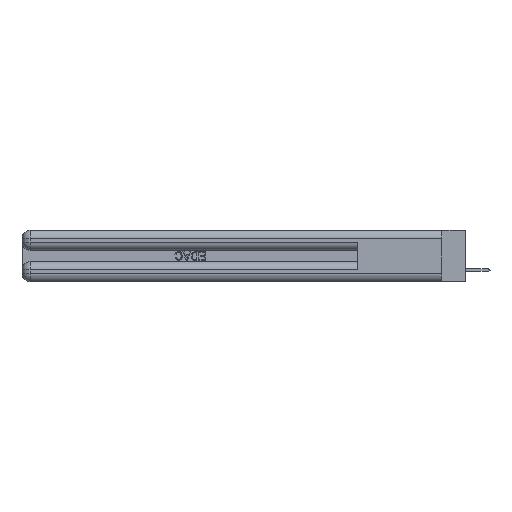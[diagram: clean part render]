
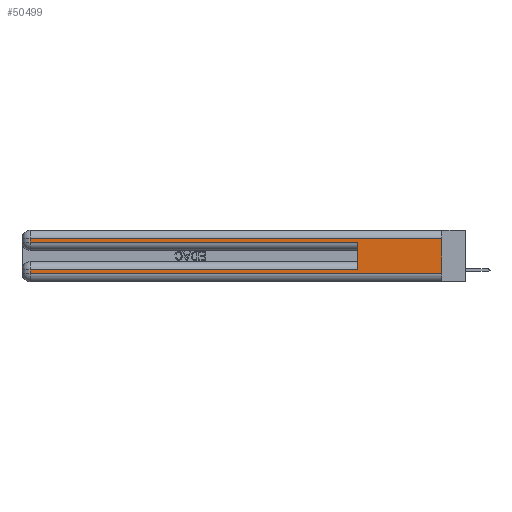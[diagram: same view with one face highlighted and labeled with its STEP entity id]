
A CAD part, left-side view. The second image highlights one B-rep face of the part: STEP entity #50499.
In plain terms, the highlighted planar face has unit normal (-1, 0, 0).
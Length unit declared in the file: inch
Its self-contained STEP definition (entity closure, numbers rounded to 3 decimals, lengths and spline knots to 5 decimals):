
#17 = VERTEX_POINT ( 'NONE', #5353 ) ;
#287 = ORIENTED_EDGE ( 'NONE', *, *, #42002, .F. ) ;
#535 = VERTEX_POINT ( 'NONE', #31533 ) ;
#2198 = LINE ( 'NONE', #14861, #20465 ) ;
#2404 = CARTESIAN_POINT ( 'NONE',  ( 0., 0., 0.085 ) ) ;
#4892 = VERTEX_POINT ( 'NONE', #27920 ) ;
#4934 = DIRECTION ( 'NONE',  ( 0., 0., -1. ) ) ;
#5353 = CARTESIAN_POINT ( 'NONE',  ( 0., 0., 0.06 ) ) ;
#5514 = VERTEX_POINT ( 'NONE', #54072 ) ;
#6959 = ORIENTED_EDGE ( 'NONE', *, *, #43028, .T. ) ;
#10789 = EDGE_LOOP ( 'NONE', ( #21644, #6959, #55105, #14437, #287, #46949, #38121, #38533 ) ) ;
#11536 = LINE ( 'NONE', #20924, #44386 ) ;
#11711 = CARTESIAN_POINT ( 'NONE',  ( 0., 2.94, 0.37 ) ) ;
#11777 = LINE ( 'NONE', #22407, #24564 ) ;
#12749 = DIRECTION ( 'NONE',  ( 0., 0., -1. ) ) ;
#14437 = ORIENTED_EDGE ( 'NONE', *, *, #19568, .T. ) ;
#14861 = CARTESIAN_POINT ( 'NONE',  ( 0., 0., 0.285 ) ) ;
#15808 = DIRECTION ( 'NONE',  ( 0., -1., 0. ) ) ;
#15972 = DIRECTION ( 'NONE',  ( 0., 1., 0. ) ) ;
#16787 = FACE_OUTER_BOUND ( 'NONE', #10789, .T. ) ;
#18270 = DIRECTION ( 'NONE',  ( 0., 0., -1. ) ) ;
#18973 = CARTESIAN_POINT ( 'NONE',  ( 0., 2.94, 0.31 ) ) ;
#19426 = VECTOR ( 'NONE', #15972, 39.37008 ) ;
#19568 = EDGE_CURVE ( 'NONE', #535, #21122, #2198, .T. ) ;
#20465 = VECTOR ( 'NONE', #48636, 39.37008 ) ;
#20551 = VECTOR ( 'NONE', #25330, 39.37008 ) ;
#20924 = CARTESIAN_POINT ( 'NONE',  ( 0., 0., 0.31 ) ) ;
#21122 = VERTEX_POINT ( 'NONE', #42955 ) ;
#21644 = ORIENTED_EDGE ( 'NONE', *, *, #52782, .F. ) ;
#22407 = CARTESIAN_POINT ( 'NONE',  ( 0., 2.94, 0.37 ) ) ;
#24564 = VECTOR ( 'NONE', #4934, 39.37008 ) ;
#25330 = DIRECTION ( 'NONE',  ( 0., 0., 1. ) ) ;
#25727 = EDGE_CURVE ( 'NONE', #29845, #5514, #48315, .T. ) ;
#26022 = CARTESIAN_POINT ( 'NONE',  ( 0., 0.6, 0.145 ) ) ;
#27412 = CARTESIAN_POINT ( 'NONE',  ( 0., 0., 0.06 ) ) ;
#27920 = CARTESIAN_POINT ( 'NONE',  ( 0., 0., 0.31 ) ) ;
#28624 = EDGE_CURVE ( 'NONE', #46204, #535, #11777, .T. ) ;
#29845 = VERTEX_POINT ( 'NONE', #52179 ) ;
#30159 = CARTESIAN_POINT ( 'NONE',  ( 0., 0., 0.37 ) ) ;
#31533 = CARTESIAN_POINT ( 'NONE',  ( 0., 2.94, 0.285 ) ) ;
#32425 = EDGE_CURVE ( 'NONE', #5514, #51431, #45002, .T. ) ;
#34370 = DIRECTION ( 'NONE',  ( 1., 0., 0. ) ) ;
#38109 = CARTESIAN_POINT ( 'NONE',  ( 0., 2.94, 0.06 ) ) ;
#38121 = ORIENTED_EDGE ( 'NONE', *, *, #32425, .T. ) ;
#38533 = ORIENTED_EDGE ( 'NONE', *, *, #50223, .T. ) ;
#39358 = CARTESIAN_POINT ( 'NONE',  ( 0., 0., 0.37 ) ) ;
#41013 = VECTOR ( 'NONE', #18270, 39.37008 ) ;
#42002 = EDGE_CURVE ( 'NONE', #29845, #21122, #46716, .T. ) ;
#42721 = LINE ( 'NONE', #30159, #52005 ) ;
#42955 = CARTESIAN_POINT ( 'NONE',  ( 0., 0.6, 0.285 ) ) ;
#43028 = EDGE_CURVE ( 'NONE', #4892, #46204, #11536, .T. ) ;
#44386 = VECTOR ( 'NONE', #55234, 39.37008 ) ;
#44973 = LINE ( 'NONE', #27412, #48331 ) ;
#45002 = LINE ( 'NONE', #11711, #41013 ) ;
#46204 = VERTEX_POINT ( 'NONE', #18973 ) ;
#46716 = LINE ( 'NONE', #26022, #20551 ) ;
#46949 = ORIENTED_EDGE ( 'NONE', *, *, #25727, .T. ) ;
#48315 = LINE ( 'NONE', #2404, #19426 ) ;
#48331 = VECTOR ( 'NONE', #15808, 39.37008 ) ;
#48636 = DIRECTION ( 'NONE',  ( 0., -1., 0. ) ) ;
#50223 = EDGE_CURVE ( 'NONE', #51431, #17, #44973, .T. ) ;
#50499 = ADVANCED_FACE ( 'NONE', ( #16787 ), #51235, .F. ) ;
#51235 = PLANE ( 'NONE',  #53751 ) ;
#51431 = VERTEX_POINT ( 'NONE', #38109 ) ;
#51948 = DIRECTION ( 'NONE',  ( 0., 0., -1. ) ) ;
#52005 = VECTOR ( 'NONE', #12749, 39.37008 ) ;
#52179 = CARTESIAN_POINT ( 'NONE',  ( 0., 0.6, 0.085 ) ) ;
#52782 = EDGE_CURVE ( 'NONE', #4892, #17, #42721, .T. ) ;
#53751 = AXIS2_PLACEMENT_3D ( 'NONE', #39358, #34370, #51948 ) ;
#54072 = CARTESIAN_POINT ( 'NONE',  ( 0., 2.94, 0.085 ) ) ;
#55105 = ORIENTED_EDGE ( 'NONE', *, *, #28624, .T. ) ;
#55234 = DIRECTION ( 'NONE',  ( 0., 1., 0. ) ) ;
